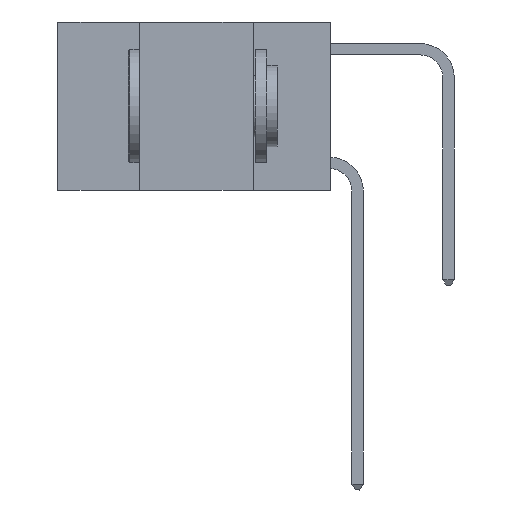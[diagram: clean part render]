
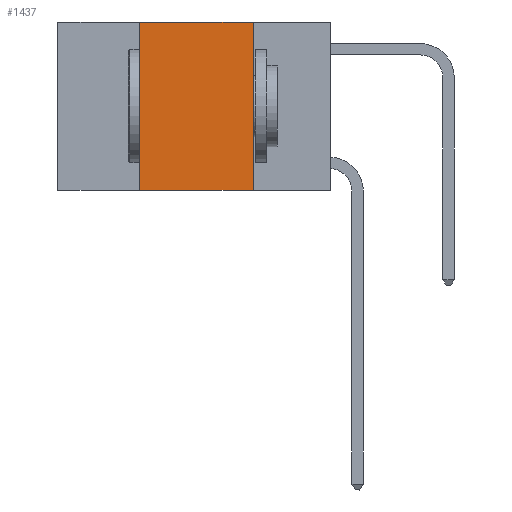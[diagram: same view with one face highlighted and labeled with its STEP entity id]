
A CAD part, left-side view. The second image highlights one B-rep face of the part: STEP entity #1437.
In plain terms, the highlighted planar face has unit normal (-1, 0, 0).
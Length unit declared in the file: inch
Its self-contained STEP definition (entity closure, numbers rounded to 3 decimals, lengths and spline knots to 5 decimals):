
#153 = EDGE_CURVE ( 'NONE', #7538, #10149, #16397, .T. ) ;
#1016 = PLANE ( 'NONE',  #14499 ) ;
#1206 = CARTESIAN_POINT ( 'NONE',  ( 0., 0.17, 0. ) ) ;
#1348 = LINE ( 'NONE', #3936, #8081 ) ;
#1384 = EDGE_CURVE ( 'NONE', #14040, #14363, #3436, .T. ) ;
#1437 = ADVANCED_FACE ( 'NONE', ( #5004 ), #1016, .F. ) ;
#3436 = LINE ( 'NONE', #10078, #12020 ) ;
#3827 = VECTOR ( 'NONE', #9898, 39.37008 ) ;
#3882 = EDGE_LOOP ( 'NONE', ( #11398, #8042, #10681, #4753 ) ) ;
#3936 = CARTESIAN_POINT ( 'NONE',  ( 0., 0.6, -0.37 ) ) ;
#4465 = LINE ( 'NONE', #6881, #13680 ) ;
#4525 = CARTESIAN_POINT ( 'NONE',  ( 0., 0.42, -0.37 ) ) ;
#4659 = CARTESIAN_POINT ( 'NONE',  ( 0., 0.17, 0. ) ) ;
#4753 = ORIENTED_EDGE ( 'NONE', *, *, #16014, .T. ) ;
#5004 = FACE_OUTER_BOUND ( 'NONE', #3882, .T. ) ;
#6295 = CARTESIAN_POINT ( 'NONE',  ( 0., 0.6, 0. ) ) ;
#6413 = DIRECTION ( 'NONE',  ( 0., 0., -1. ) ) ;
#6881 = CARTESIAN_POINT ( 'NONE',  ( 0., 0.6, 0. ) ) ;
#7538 = VERTEX_POINT ( 'NONE', #1206 ) ;
#8042 = ORIENTED_EDGE ( 'NONE', *, *, #9327, .F. ) ;
#8081 = VECTOR ( 'NONE', #9179, 39.37008 ) ;
#8686 = DIRECTION ( 'NONE',  ( 0., 0., 1. ) ) ;
#9179 = DIRECTION ( 'NONE',  ( 0., -1., 0. ) ) ;
#9327 = EDGE_CURVE ( 'NONE', #14363, #7538, #4465, .T. ) ;
#9898 = DIRECTION ( 'NONE',  ( 0., 0., -1. ) ) ;
#10078 = CARTESIAN_POINT ( 'NONE',  ( 0., 0.42, 0. ) ) ;
#10149 = VERTEX_POINT ( 'NONE', #12290 ) ;
#10681 = ORIENTED_EDGE ( 'NONE', *, *, #1384, .F. ) ;
#11398 = ORIENTED_EDGE ( 'NONE', *, *, #153, .F. ) ;
#12020 = VECTOR ( 'NONE', #8686, 39.37008 ) ;
#12265 = DIRECTION ( 'NONE',  ( 0., -1., 0. ) ) ;
#12290 = CARTESIAN_POINT ( 'NONE',  ( 0., 0.17, -0.37 ) ) ;
#13680 = VECTOR ( 'NONE', #12265, 39.37008 ) ;
#14040 = VERTEX_POINT ( 'NONE', #4525 ) ;
#14304 = CARTESIAN_POINT ( 'NONE',  ( 0., 0.42, 0. ) ) ;
#14363 = VERTEX_POINT ( 'NONE', #14304 ) ;
#14499 = AXIS2_PLACEMENT_3D ( 'NONE', #6295, #16736, #6413 ) ;
#16014 = EDGE_CURVE ( 'NONE', #14040, #10149, #1348, .T. ) ;
#16397 = LINE ( 'NONE', #4659, #3827 ) ;
#16736 = DIRECTION ( 'NONE',  ( 1., 0., 0. ) ) ;
